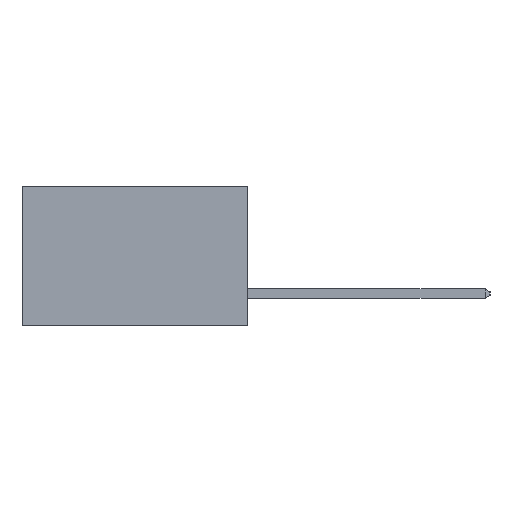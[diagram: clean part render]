
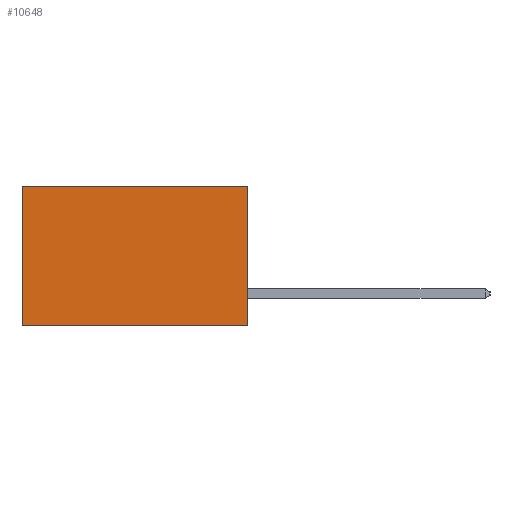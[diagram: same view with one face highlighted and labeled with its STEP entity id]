
A CAD part, left-side view. The second image highlights one B-rep face of the part: STEP entity #10648.
In plain terms, the highlighted planar face has unit normal (-1, 0, 0).
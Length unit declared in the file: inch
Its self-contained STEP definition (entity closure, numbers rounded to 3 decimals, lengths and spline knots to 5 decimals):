
#47 = LINE ( 'NONE', #142, #10178 ) ;
#142 = CARTESIAN_POINT ( 'NONE',  ( 0.2615, 0., -0.37 ) ) ;
#171 = ORIENTED_EDGE ( 'NONE', *, *, #3517, .F. ) ;
#519 = CARTESIAN_POINT ( 'NONE',  ( 0.2615, 0., 0. ) ) ;
#1606 = CARTESIAN_POINT ( 'NONE',  ( 0.2615, 0.6, 0. ) ) ;
#2317 = LINE ( 'NONE', #519, #9289 ) ;
#2466 = DIRECTION ( 'NONE',  ( 0., 1., 0. ) ) ;
#2784 = EDGE_CURVE ( 'NONE', #3148, #12153, #3516, .T. ) ;
#3035 = ORIENTED_EDGE ( 'NONE', *, *, #3165, .F. ) ;
#3048 = ORIENTED_EDGE ( 'NONE', *, *, #4710, .T. ) ;
#3148 = VERTEX_POINT ( 'NONE', #1606 ) ;
#3165 = EDGE_CURVE ( 'NONE', #8708, #12153, #47, .T. ) ;
#3172 = VECTOR ( 'NONE', #7943, 39.37008 ) ;
#3233 = CARTESIAN_POINT ( 'NONE',  ( 0.2615, 0., -0.37 ) ) ;
#3516 = LINE ( 'NONE', #8056, #3172 ) ;
#3517 = EDGE_CURVE ( 'NONE', #9841, #8708, #11119, .T. ) ;
#3970 = DIRECTION ( 'NONE',  ( 0., 0., -1. ) ) ;
#4243 = DIRECTION ( 'NONE',  ( 1., 0., 0. ) ) ;
#4710 = EDGE_CURVE ( 'NONE', #9841, #3148, #2317, .T. ) ;
#4906 = CARTESIAN_POINT ( 'NONE',  ( 0.2615, 0., -0.37 ) ) ;
#5031 = AXIS2_PLACEMENT_3D ( 'NONE', #3233, #4243, #10590 ) ;
#5685 = CARTESIAN_POINT ( 'NONE',  ( 0.2615, 0.6, -0.37 ) ) ;
#6711 = DIRECTION ( 'NONE',  ( 0., 1., 0. ) ) ;
#6979 = FACE_OUTER_BOUND ( 'NONE', #8394, .T. ) ;
#7943 = DIRECTION ( 'NONE',  ( 0., 0., -1. ) ) ;
#8056 = CARTESIAN_POINT ( 'NONE',  ( 0.2615, 0.6, -0.37 ) ) ;
#8205 = VECTOR ( 'NONE', #3970, 39.37008 ) ;
#8394 = EDGE_LOOP ( 'NONE', ( #8987, #3035, #171, #3048 ) ) ;
#8708 = VERTEX_POINT ( 'NONE', #9544 ) ;
#8809 = PLANE ( 'NONE',  #5031 ) ;
#8987 = ORIENTED_EDGE ( 'NONE', *, *, #2784, .T. ) ;
#9289 = VECTOR ( 'NONE', #6711, 39.37008 ) ;
#9544 = CARTESIAN_POINT ( 'NONE',  ( 0.2615, 0., -0.37 ) ) ;
#9841 = VERTEX_POINT ( 'NONE', #11395 ) ;
#10178 = VECTOR ( 'NONE', #2466, 39.37008 ) ;
#10590 = DIRECTION ( 'NONE',  ( 0., 0., -1. ) ) ;
#10648 = ADVANCED_FACE ( 'NONE', ( #6979 ), #8809, .F. ) ;
#11119 = LINE ( 'NONE', #4906, #8205 ) ;
#11395 = CARTESIAN_POINT ( 'NONE',  ( 0.2615, 0., 0. ) ) ;
#12153 = VERTEX_POINT ( 'NONE', #5685 ) ;
